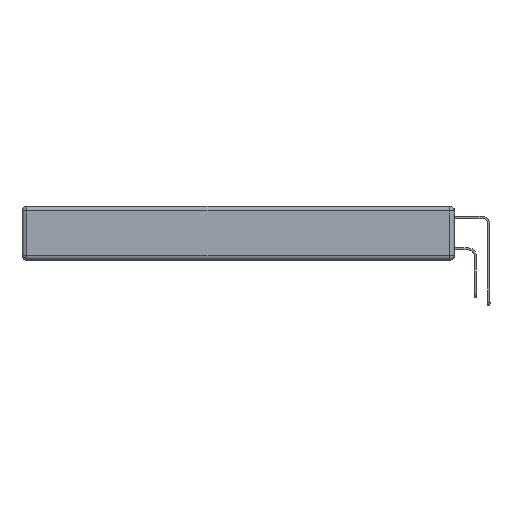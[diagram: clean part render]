
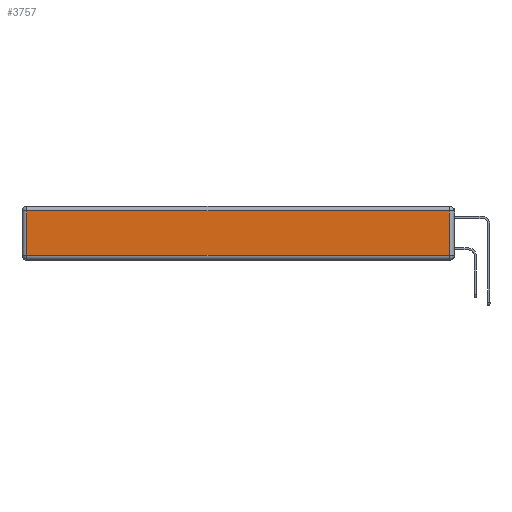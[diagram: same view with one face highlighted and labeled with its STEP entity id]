
A CAD part, left-side view. The second image highlights one B-rep face of the part: STEP entity #3757.
In plain terms, the highlighted planar face has unit normal (-1, 0, 0).
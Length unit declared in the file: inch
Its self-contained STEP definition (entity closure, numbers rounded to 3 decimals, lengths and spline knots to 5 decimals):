
#200 = DIRECTION ( 'NONE',  ( 0., 0., 1. ) ) ;
#990 = EDGE_CURVE ( 'NONE', #4156, #2032, #1699, .T. ) ;
#1699 = LINE ( 'NONE', #13940, #16724 ) ;
#1839 = FACE_OUTER_BOUND ( 'NONE', #8800, .T. ) ;
#2032 = VERTEX_POINT ( 'NONE', #11964 ) ;
#2075 = VERTEX_POINT ( 'NONE', #17577 ) ;
#3362 = LINE ( 'NONE', #5874, #13159 ) ;
#3757 = ADVANCED_FACE ( 'NONE', ( #1839 ), #4724, .T. ) ;
#4156 = VERTEX_POINT ( 'NONE', #14154 ) ;
#4272 = ORIENTED_EDGE ( 'NONE', *, *, #990, .T. ) ;
#4724 = PLANE ( 'NONE',  #7040 ) ;
#5175 = DIRECTION ( 'NONE',  ( 0., 1., 0. ) ) ;
#5208 = CARTESIAN_POINT ( 'NONE',  ( 0., 0., -0.313 ) ) ;
#5874 = CARTESIAN_POINT ( 'NONE',  ( 0., 2.72, -0.343 ) ) ;
#6167 = VECTOR ( 'NONE', #5175, 39.37008 ) ;
#7040 = AXIS2_PLACEMENT_3D ( 'NONE', #7332, #12817, #200 ) ;
#7284 = VERTEX_POINT ( 'NONE', #11070 ) ;
#7332 = CARTESIAN_POINT ( 'NONE',  ( 0., 0., -0.343 ) ) ;
#8800 = EDGE_LOOP ( 'NONE', ( #15695, #4272, #16690, #16914 ) ) ;
#10275 = DIRECTION ( 'NONE',  ( 0., 0., -1. ) ) ;
#10595 = EDGE_CURVE ( 'NONE', #2075, #4156, #12047, .T. ) ;
#10695 = DIRECTION ( 'NONE',  ( 0., -1., 0. ) ) ;
#11036 = EDGE_CURVE ( 'NONE', #2032, #7284, #12106, .T. ) ;
#11070 = CARTESIAN_POINT ( 'NONE',  ( 0., 2.72, -0.03 ) ) ;
#11244 = DIRECTION ( 'NONE',  ( 0., 0., 1. ) ) ;
#11807 = VECTOR ( 'NONE', #10695, 39.37008 ) ;
#11964 = CARTESIAN_POINT ( 'NONE',  ( 0., 0.03, -0.03 ) ) ;
#12047 = LINE ( 'NONE', #5208, #11807 ) ;
#12106 = LINE ( 'NONE', #16103, #6167 ) ;
#12817 = DIRECTION ( 'NONE',  ( -1., 0., 0. ) ) ;
#13159 = VECTOR ( 'NONE', #10275, 39.37008 ) ;
#13281 = EDGE_CURVE ( 'NONE', #7284, #2075, #3362, .T. ) ;
#13940 = CARTESIAN_POINT ( 'NONE',  ( 0., 0.03, -0.343 ) ) ;
#14154 = CARTESIAN_POINT ( 'NONE',  ( 0., 0.03, -0.313 ) ) ;
#15695 = ORIENTED_EDGE ( 'NONE', *, *, #10595, .T. ) ;
#16103 = CARTESIAN_POINT ( 'NONE',  ( 0., 2.75, -0.03 ) ) ;
#16690 = ORIENTED_EDGE ( 'NONE', *, *, #11036, .T. ) ;
#16724 = VECTOR ( 'NONE', #11244, 39.37008 ) ;
#16914 = ORIENTED_EDGE ( 'NONE', *, *, #13281, .T. ) ;
#17577 = CARTESIAN_POINT ( 'NONE',  ( 0., 2.72, -0.313 ) ) ;
